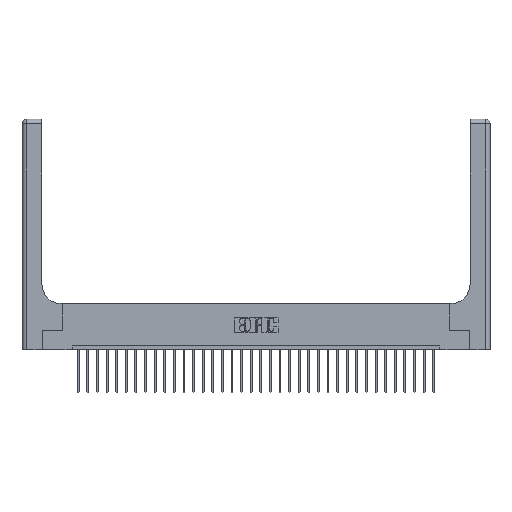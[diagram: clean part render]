
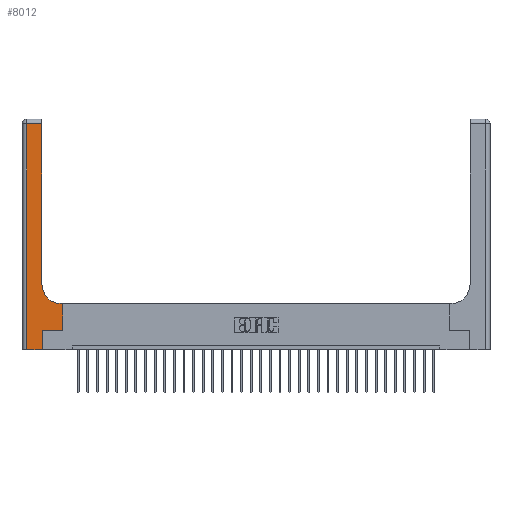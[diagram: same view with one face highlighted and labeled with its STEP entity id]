
A CAD part, top view. The second image highlights one B-rep face of the part: STEP entity #8012.
In plain terms, the highlighted planar face has unit normal (0, 0, 1).
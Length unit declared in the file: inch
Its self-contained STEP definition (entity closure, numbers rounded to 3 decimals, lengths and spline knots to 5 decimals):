
#281 = LINE ( 'NONE', #23616, #19900 ) ;
#354 = LINE ( 'NONE', #25482, #10300 ) ;
#430 = EDGE_CURVE ( 'NONE', #15237, #18414, #3461, .T. ) ;
#503 = ORIENTED_EDGE ( 'NONE', *, *, #13918, .T. ) ;
#742 = DIRECTION ( 'NONE',  ( -1., 0., 0. ) ) ;
#753 = ORIENTED_EDGE ( 'NONE', *, *, #6180, .T. ) ;
#1049 = DIRECTION ( 'NONE',  ( 0., 1., 0. ) ) ;
#3011 = PLANE ( 'NONE',  #15641 ) ;
#3461 = LINE ( 'NONE', #8128, #4240 ) ;
#3874 = EDGE_CURVE ( 'NONE', #24071, #15237, #28122, .T. ) ;
#4022 = ORIENTED_EDGE ( 'NONE', *, *, #10832, .T. ) ;
#4240 = VECTOR ( 'NONE', #10389, 39.37008 ) ;
#4465 = CARTESIAN_POINT ( 'NONE',  ( 0.26, 0.85, 0.37 ) ) ;
#4658 = EDGE_CURVE ( 'NONE', #22593, #24071, #13189, .T. ) ;
#5178 = CARTESIAN_POINT ( 'NONE',  ( 0.265, 0.25, 0.37 ) ) ;
#5405 = CARTESIAN_POINT ( 'NONE',  ( 0.51, 0.6, 0.37 ) ) ;
#5632 = CARTESIAN_POINT ( 'NONE',  ( 0.265, 0., 0.37 ) ) ;
#6180 = EDGE_CURVE ( 'NONE', #23817, #11137, #354, .T. ) ;
#6548 = CARTESIAN_POINT ( 'NONE',  ( 0.06, 0., 0.37 ) ) ;
#6750 = VECTOR ( 'NONE', #22401, 39.37008 ) ;
#8012 = ADVANCED_FACE ( 'NONE', ( #23612 ), #3011, .F. ) ;
#8026 = ORIENTED_EDGE ( 'NONE', *, *, #26178, .T. ) ;
#8128 = CARTESIAN_POINT ( 'NONE',  ( 0., 0., 0.37 ) ) ;
#8543 = ORIENTED_EDGE ( 'NONE', *, *, #19915, .T. ) ;
#9941 = CARTESIAN_POINT ( 'NONE',  ( 0.06, 3., 0.37 ) ) ;
#10300 = VECTOR ( 'NONE', #25941, 39.37008 ) ;
#10389 = DIRECTION ( 'NONE',  ( 1., 0., 0. ) ) ;
#10401 = CARTESIAN_POINT ( 'NONE',  ( 0.528, 0.25, 0.37 ) ) ;
#10832 = EDGE_CURVE ( 'NONE', #26290, #23817, #26922, .T. ) ;
#11137 = VERTEX_POINT ( 'NONE', #5405 ) ;
#11332 = EDGE_LOOP ( 'NONE', ( #8543, #25783, #27949, #27644, #8026, #19407, #4022, #753, #503 ) ) ;
#11373 = VECTOR ( 'NONE', #1049, 39.37008 ) ;
#11447 = CARTESIAN_POINT ( 'NONE',  ( 0.265, 0.25, 0.37 ) ) ;
#13148 = VECTOR ( 'NONE', #14123, 39.37008 ) ;
#13189 = LINE ( 'NONE', #22350, #19397 ) ;
#13918 = EDGE_CURVE ( 'NONE', #11137, #18760, #28310, .T. ) ;
#14123 = DIRECTION ( 'NONE',  ( 0., -1., 0. ) ) ;
#14363 = AXIS2_PLACEMENT_3D ( 'NONE', #24596, #18934, #19942 ) ;
#14489 = LINE ( 'NONE', #5178, #24530 ) ;
#15040 = LINE ( 'NONE', #24068, #6750 ) ;
#15151 = CARTESIAN_POINT ( 'NONE',  ( 0.528, 0.6, 0.37 ) ) ;
#15237 = VERTEX_POINT ( 'NONE', #6548 ) ;
#15462 = EDGE_CURVE ( 'NONE', #29147, #26290, #14489, .T. ) ;
#15641 = AXIS2_PLACEMENT_3D ( 'NONE', #21360, #18784, #742 ) ;
#18414 = VERTEX_POINT ( 'NONE', #5632 ) ;
#18760 = VERTEX_POINT ( 'NONE', #4465 ) ;
#18784 = DIRECTION ( 'NONE',  ( 0., 0., -1. ) ) ;
#18934 = DIRECTION ( 'NONE',  ( 0., 0., -1. ) ) ;
#19397 = VECTOR ( 'NONE', #27009, 39.37008 ) ;
#19407 = ORIENTED_EDGE ( 'NONE', *, *, #15462, .T. ) ;
#19445 = DIRECTION ( 'NONE',  ( 1., 0., 0. ) ) ;
#19900 = VECTOR ( 'NONE', #28130, 39.37008 ) ;
#19915 = EDGE_CURVE ( 'NONE', #18760, #22593, #15040, .T. ) ;
#19942 = DIRECTION ( 'NONE',  ( 1., 0., 0. ) ) ;
#21360 = CARTESIAN_POINT ( 'NONE',  ( 0., 3., 0.37 ) ) ;
#21492 = CARTESIAN_POINT ( 'NONE',  ( 0.528, 0.25, 0.37 ) ) ;
#22350 = CARTESIAN_POINT ( 'NONE',  ( 0., 2.94, 0.37 ) ) ;
#22401 = DIRECTION ( 'NONE',  ( 0., 1., 0. ) ) ;
#22593 = VERTEX_POINT ( 'NONE', #26761 ) ;
#23612 = FACE_OUTER_BOUND ( 'NONE', #11332, .T. ) ;
#23616 = CARTESIAN_POINT ( 'NONE',  ( 0.265, 0., 0.37 ) ) ;
#23817 = VERTEX_POINT ( 'NONE', #15151 ) ;
#24068 = CARTESIAN_POINT ( 'NONE',  ( 0.26, 3., 0.37 ) ) ;
#24071 = VERTEX_POINT ( 'NONE', #29725 ) ;
#24530 = VECTOR ( 'NONE', #19445, 39.37008 ) ;
#24596 = CARTESIAN_POINT ( 'NONE',  ( 0.51, 0.85, 0.37 ) ) ;
#25482 = CARTESIAN_POINT ( 'NONE',  ( 0.26, 0.6, 0.37 ) ) ;
#25783 = ORIENTED_EDGE ( 'NONE', *, *, #4658, .T. ) ;
#25941 = DIRECTION ( 'NONE',  ( -1., 0., 0. ) ) ;
#26178 = EDGE_CURVE ( 'NONE', #18414, #29147, #281, .T. ) ;
#26290 = VERTEX_POINT ( 'NONE', #21492 ) ;
#26761 = CARTESIAN_POINT ( 'NONE',  ( 0.26, 2.94, 0.37 ) ) ;
#26922 = LINE ( 'NONE', #10401, #11373 ) ;
#27009 = DIRECTION ( 'NONE',  ( -1., 0., 0. ) ) ;
#27644 = ORIENTED_EDGE ( 'NONE', *, *, #430, .T. ) ;
#27949 = ORIENTED_EDGE ( 'NONE', *, *, #3874, .T. ) ;
#28122 = LINE ( 'NONE', #9941, #13148 ) ;
#28130 = DIRECTION ( 'NONE',  ( 0., 1., 0. ) ) ;
#28310 = CIRCLE ( 'NONE', #14363, 0.25 ) ;
#29147 = VERTEX_POINT ( 'NONE', #11447 ) ;
#29725 = CARTESIAN_POINT ( 'NONE',  ( 0.06, 2.94, 0.37 ) ) ;
